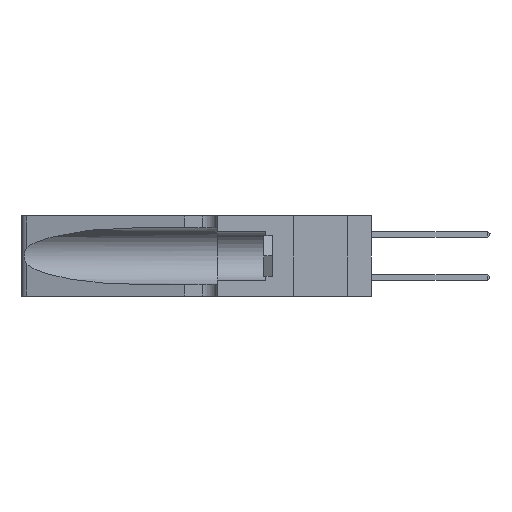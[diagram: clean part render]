
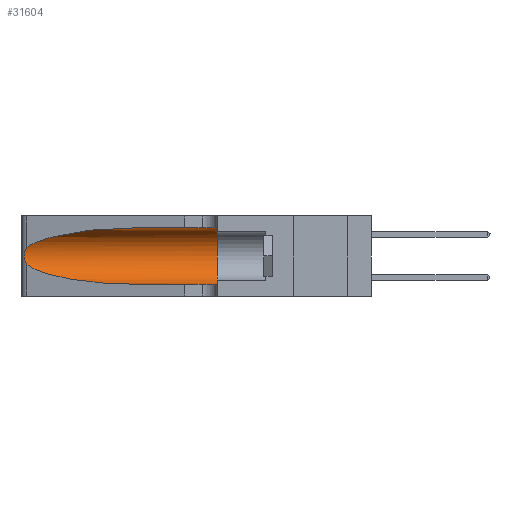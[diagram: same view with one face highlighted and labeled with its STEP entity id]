
A CAD part, left-side view. The second image highlights one B-rep face of the part: STEP entity #31604.
In plain terms, the highlighted cylindrical face has radius 3.308 mm (diameter 6.617 mm), a partial arc.
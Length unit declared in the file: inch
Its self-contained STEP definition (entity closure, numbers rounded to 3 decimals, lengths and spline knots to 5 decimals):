
#507 = CARTESIAN_POINT ( 'NONE',  ( 0.25856, 1.23593, 0.16098 ) ) ;
#1332 = CARTESIAN_POINT ( 'NONE',  ( 0.1305, 0.72297, 0.05475 ) ) ;
#1438 = CARTESIAN_POINT ( 'NONE',  ( 0.25487, 1.22718, 0.22369 ) ) ;
#1580 = VERTEX_POINT ( 'NONE', #9592 ) ;
#3523 = EDGE_LOOP ( 'NONE', ( #29691, #24228, #33425, #23249, #32425, #38322 ) ) ;
#5141 = DIRECTION ( 'NONE',  ( 0., 0., 1. ) ) ;
#5164 = CARTESIAN_POINT ( 'NONE',  ( 0.1305, 1.61858, 0.31525 ) ) ;
#6228 = CARTESIAN_POINT ( 'NONE',  ( 0.25555, 1.22994, 0.2215 ) ) ;
#6306 = DIRECTION ( 'NONE',  ( 0., 0., -1. ) ) ;
#6336 = VERTEX_POINT ( 'NONE', #16467 ) ;
#6863 = CARTESIAN_POINT ( 'NONE',  ( 0.26075, 1.23896, 0.178 ) ) ;
#7187 = VERTEX_POINT ( 'NONE', #15835 ) ;
#8950 =( BOUNDED_CURVE ( )  B_SPLINE_CURVE ( 3, ( #33995, #18751, #31070, #24742 ),
 .UNSPECIFIED., .F., .F. ) 
 B_SPLINE_CURVE_WITH_KNOTS ( ( 4, 4 ),
 ( 1.5708, 2.84003 ),
 .UNSPECIFIED. ) 
 CURVE ( )  GEOMETRIC_REPRESENTATION_ITEM ( )  RATIONAL_B_SPLINE_CURVE ( ( 1., 0.87, 0.87, 1. ) ) 
 REPRESENTATION_ITEM ( '' )  );
#9592 = CARTESIAN_POINT ( 'NONE',  ( 0.1305, 0.35, 0.31525 ) ) ;
#9665 = CARTESIAN_POINT ( 'NONE',  ( 0.25639, 1.23186, 0.15144 ) ) ;
#9788 = CARTESIAN_POINT ( 'NONE',  ( 0.26075, 1.23896, 0.19203 ) ) ;
#10959 = CARTESIAN_POINT ( 'NONE',  ( 0.1305, 0.35, 0.185 ) ) ;
#11354 =( BOUNDED_CURVE ( )  B_SPLINE_CURVE ( 3, ( #32642, #17550, #14644, #17687 ),
 .UNSPECIFIED., .F., .T. ) 
 B_SPLINE_CURVE_WITH_KNOTS ( ( 4, 4 ),
 ( 3.44316, 4.71239 ),
 .UNSPECIFIED. ) 
 CURVE ( )  GEOMETRIC_REPRESENTATION_ITEM ( )  RATIONAL_B_SPLINE_CURVE ( ( 1., 0.87, 0.87, 1. ) ) 
 REPRESENTATION_ITEM ( '' )  );
#13079 = CARTESIAN_POINT ( 'NONE',  ( 0.26017, 1.23833, 0.17102 ) ) ;
#13532 = EDGE_CURVE ( 'NONE', #1580, #6336, #25322, .T. ) ;
#14532 = LINE ( 'NONE', #5164, #24017 ) ;
#14644 = CARTESIAN_POINT ( 'NONE',  ( 0.18966, 0.96281, 0.05475 ) ) ;
#14900 = LINE ( 'NONE', #25235, #29162 ) ;
#15177 = DIRECTION ( 'NONE',  ( 0., -1., 0. ) ) ;
#15835 = CARTESIAN_POINT ( 'NONE',  ( 0.25487, 1.22718, 0.14631 ) ) ;
#16019 = CYLINDRICAL_SURFACE ( 'NONE', #31271, 0.13025 ) ;
#16467 = CARTESIAN_POINT ( 'NONE',  ( 0.1305, 0.35, 0.05475 ) ) ;
#17550 = CARTESIAN_POINT ( 'NONE',  ( 0.2373, 1.15595, 0.08982 ) ) ;
#17687 = CARTESIAN_POINT ( 'NONE',  ( 0.1305, 0.72297, 0.05475 ) ) ;
#18552 = EDGE_CURVE ( 'NONE', #37642, #1580, #14532, .T. ) ;
#18751 = CARTESIAN_POINT ( 'NONE',  ( 0.18966, 0.96281, 0.31525 ) ) ;
#18871 = FACE_OUTER_BOUND ( 'NONE', #3523, .T. ) ;
#18922 = CARTESIAN_POINT ( 'NONE',  ( 0.25555, 1.22993, 0.14849 ) ) ;
#19513 = DIRECTION ( 'NONE',  ( 0., -1., 0. ) ) ;
#20226 = VERTEX_POINT ( 'NONE', #1438 ) ;
#20242 = DIRECTION ( 'NONE',  ( 0., 1., 0. ) ) ;
#21051 = DIRECTION ( 'NONE',  ( 0., -1., 0. ) ) ;
#22103 = CARTESIAN_POINT ( 'NONE',  ( 0.25487, 1.22718, 0.14631 ) ) ;
#23249 = ORIENTED_EDGE ( 'NONE', *, *, #33982, .T. ) ;
#24011 = EDGE_CURVE ( 'NONE', #20226, #7187, #24255, .T. ) ;
#24017 = VECTOR ( 'NONE', #21051, 39.37008 ) ;
#24228 = ORIENTED_EDGE ( 'NONE', *, *, #24011, .T. ) ;
#24255 = B_SPLINE_CURVE_WITH_KNOTS ( 'NONE', 3,
 ( #24401, #6228, #37205, #30722, #36814, #34304, #9788, #6863, #13079, #507, #28117, #9665, #18922, #22103 ),
 .UNSPECIFIED., .F., .F.,
 ( 4, 2, 2, 2, 2, 2, 4 ),
 ( 0., 0.00027, 0.00053, 0.00107, 0.0016, 0.00187, 0.00214 ),
 .UNSPECIFIED. ) ;
#24401 = CARTESIAN_POINT ( 'NONE',  ( 0.25487, 1.22718, 0.22369 ) ) ;
#24742 = CARTESIAN_POINT ( 'NONE',  ( 0.25487, 1.22718, 0.22369 ) ) ;
#25235 = CARTESIAN_POINT ( 'NONE',  ( 0.1305, 1.61858, 0.05475 ) ) ;
#25322 = CIRCLE ( 'NONE', #31416, 0.13025 ) ;
#28117 = CARTESIAN_POINT ( 'NONE',  ( 0.25789, 1.23486, 0.15765 ) ) ;
#29162 = VECTOR ( 'NONE', #19513, 39.37008 ) ;
#29691 = ORIENTED_EDGE ( 'NONE', *, *, #36976, .T. ) ;
#30160 = CARTESIAN_POINT ( 'NONE',  ( 0.1305, 1.61858, 0.185 ) ) ;
#30722 = CARTESIAN_POINT ( 'NONE',  ( 0.25787, 1.23484, 0.2124 ) ) ;
#31009 = VERTEX_POINT ( 'NONE', #1332 ) ;
#31070 = CARTESIAN_POINT ( 'NONE',  ( 0.2373, 1.15595, 0.28018 ) ) ;
#31271 = AXIS2_PLACEMENT_3D ( 'NONE', #30160, #15177, #6306 ) ;
#31416 = AXIS2_PLACEMENT_3D ( 'NONE', #10959, #20242, #5141 ) ;
#31604 = ADVANCED_FACE ( 'NONE', ( #18871 ), #16019, .F. ) ;
#32425 = ORIENTED_EDGE ( 'NONE', *, *, #13532, .F. ) ;
#32642 = CARTESIAN_POINT ( 'NONE',  ( 0.25487, 1.22718, 0.14631 ) ) ;
#33425 = ORIENTED_EDGE ( 'NONE', *, *, #35516, .T. ) ;
#33982 = EDGE_CURVE ( 'NONE', #31009, #6336, #14900, .T. ) ;
#33995 = CARTESIAN_POINT ( 'NONE',  ( 0.1305, 0.72297, 0.31525 ) ) ;
#34304 = CARTESIAN_POINT ( 'NONE',  ( 0.26018, 1.23835, 0.19895 ) ) ;
#35516 = EDGE_CURVE ( 'NONE', #7187, #31009, #11354, .T. ) ;
#36814 = CARTESIAN_POINT ( 'NONE',  ( 0.25854, 1.2359, 0.20912 ) ) ;
#36976 = EDGE_CURVE ( 'NONE', #37642, #20226, #8950, .T. ) ;
#37205 = CARTESIAN_POINT ( 'NONE',  ( 0.25639, 1.23184, 0.21858 ) ) ;
#37642 = VERTEX_POINT ( 'NONE', #37705 ) ;
#37705 = CARTESIAN_POINT ( 'NONE',  ( 0.1305, 0.72297, 0.31525 ) ) ;
#38322 = ORIENTED_EDGE ( 'NONE', *, *, #18552, .F. ) ;
